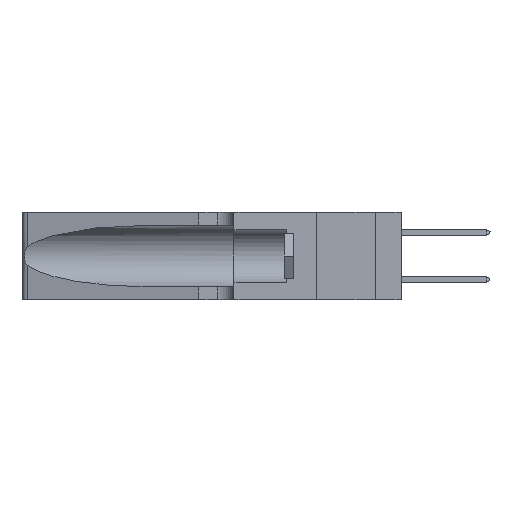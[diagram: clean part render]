
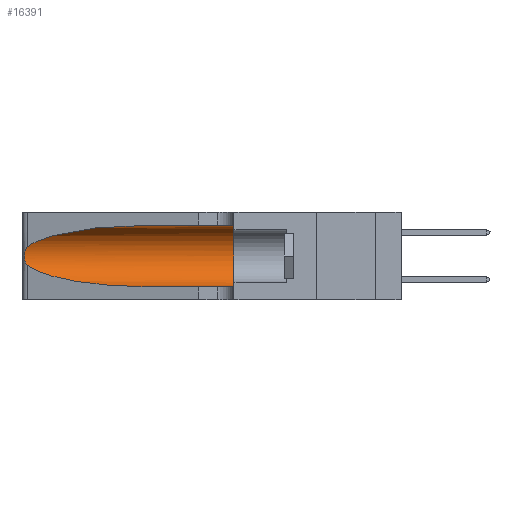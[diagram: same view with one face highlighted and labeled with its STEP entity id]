
A CAD part, left-side view. The second image highlights one B-rep face of the part: STEP entity #16391.
In plain terms, the highlighted cylindrical face has radius 3.308 mm (diameter 6.617 mm), a partial arc.
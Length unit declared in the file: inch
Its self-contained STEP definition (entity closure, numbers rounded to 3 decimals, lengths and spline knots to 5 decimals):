
#79 = DIRECTION ( 'NONE',  ( 0., 1., 0. ) ) ;
#780 = VERTEX_POINT ( 'NONE', #5503 ) ;
#1505 =( BOUNDED_CURVE ( )  B_SPLINE_CURVE ( 3, ( #8014, #35577, #5180, #27400 ),
 .UNSPECIFIED., .F., .F. ) 
 B_SPLINE_CURVE_WITH_KNOTS ( ( 4, 4 ),
 ( 1.5708, 2.84003 ),
 .UNSPECIFIED. ) 
 CURVE ( )  GEOMETRIC_REPRESENTATION_ITEM ( )  RATIONAL_B_SPLINE_CURVE ( ( 1., 0.87, 0.87, 1. ) ) 
 REPRESENTATION_ITEM ( '' )  );
#2190 = EDGE_CURVE ( 'NONE', #30342, #19642, #1505, .T. ) ;
#2523 = VERTEX_POINT ( 'NONE', #34253 ) ;
#2608 = AXIS2_PLACEMENT_3D ( 'NONE', #16649, #2687, #22255 ) ;
#2687 = DIRECTION ( 'NONE',  ( 0., -1., 0. ) ) ;
#2795 = CARTESIAN_POINT ( 'NONE',  ( 0.26075, 1.23896, 0.19203 ) ) ;
#2857 = CARTESIAN_POINT ( 'NONE',  ( 0.18966, 0.96281, 0.05475 ) ) ;
#3295 = CARTESIAN_POINT ( 'NONE',  ( 0.1305, 1.61858, 0.31525 ) ) ;
#3345 = CYLINDRICAL_SURFACE ( 'NONE', #2608, 0.13025 ) ;
#3600 = EDGE_CURVE ( 'NONE', #25010, #780, #31167, .T. ) ;
#4229 = VECTOR ( 'NONE', #25570, 39.37008 ) ;
#4769 = CARTESIAN_POINT ( 'NONE',  ( 0.1305, 0.35, 0.31525 ) ) ;
#4921 = CARTESIAN_POINT ( 'NONE',  ( 0.25854, 1.2359, 0.20912 ) ) ;
#5127 = LINE ( 'NONE', #3295, #4229 ) ;
#5180 = CARTESIAN_POINT ( 'NONE',  ( 0.2373, 1.15595, 0.28018 ) ) ;
#5503 = CARTESIAN_POINT ( 'NONE',  ( 0.1305, 0.72297, 0.05475 ) ) ;
#5655 = CARTESIAN_POINT ( 'NONE',  ( 0.26017, 1.23833, 0.17102 ) ) ;
#6719 = CARTESIAN_POINT ( 'NONE',  ( 0.1305, 1.61858, 0.05475 ) ) ;
#7642 = EDGE_CURVE ( 'NONE', #19642, #25010, #24781, .T. ) ;
#8014 = CARTESIAN_POINT ( 'NONE',  ( 0.1305, 0.72297, 0.31525 ) ) ;
#8484 = CARTESIAN_POINT ( 'NONE',  ( 0.25789, 1.23486, 0.15765 ) ) ;
#11166 = EDGE_CURVE ( 'NONE', #30342, #30793, #5127, .T. ) ;
#11323 = CARTESIAN_POINT ( 'NONE',  ( 0.25555, 1.22993, 0.14849 ) ) ;
#14020 = CARTESIAN_POINT ( 'NONE',  ( 0.25487, 1.22718, 0.14631 ) ) ;
#14827 = EDGE_LOOP ( 'NONE', ( #20320, #20358, #21930, #22823, #23377, #23722 ) ) ;
#15326 = EDGE_CURVE ( 'NONE', #780, #2523, #17873, .T. ) ;
#16123 = VECTOR ( 'NONE', #23384, 39.37008 ) ;
#16391 = ADVANCED_FACE ( 'NONE', ( #18219 ), #3345, .F. ) ;
#16649 = CARTESIAN_POINT ( 'NONE',  ( 0.1305, 1.61858, 0.185 ) ) ;
#16758 = CARTESIAN_POINT ( 'NONE',  ( 0.25787, 1.23484, 0.2124 ) ) ;
#16860 = CARTESIAN_POINT ( 'NONE',  ( 0.1305, 0.35, 0.185 ) ) ;
#17873 = LINE ( 'NONE', #6719, #16123 ) ;
#18219 = FACE_OUTER_BOUND ( 'NONE', #14827, .T. ) ;
#18977 = CARTESIAN_POINT ( 'NONE',  ( 0.25487, 1.22718, 0.14631 ) ) ;
#19562 = CARTESIAN_POINT ( 'NONE',  ( 0.26018, 1.23835, 0.19895 ) ) ;
#19642 = VERTEX_POINT ( 'NONE', #27674 ) ;
#19662 = DIRECTION ( 'NONE',  ( 0., 0., 1. ) ) ;
#19808 = CARTESIAN_POINT ( 'NONE',  ( 0.1305, 0.72297, 0.31525 ) ) ;
#20320 = ORIENTED_EDGE ( 'NONE', *, *, #2190, .T. ) ;
#20358 = ORIENTED_EDGE ( 'NONE', *, *, #7642, .T. ) ;
#21095 = AXIS2_PLACEMENT_3D ( 'NONE', #16860, #79, #19662 ) ;
#21930 = ORIENTED_EDGE ( 'NONE', *, *, #3600, .T. ) ;
#22242 = CARTESIAN_POINT ( 'NONE',  ( 0.25555, 1.22994, 0.2215 ) ) ;
#22255 = DIRECTION ( 'NONE',  ( 0., 0., -1. ) ) ;
#22353 = CARTESIAN_POINT ( 'NONE',  ( 0.26075, 1.23896, 0.178 ) ) ;
#22413 = CARTESIAN_POINT ( 'NONE',  ( 0.1305, 0.72297, 0.05475 ) ) ;
#22823 = ORIENTED_EDGE ( 'NONE', *, *, #15326, .T. ) ;
#23377 = ORIENTED_EDGE ( 'NONE', *, *, #35467, .F. ) ;
#23384 = DIRECTION ( 'NONE',  ( 0., -1., 0. ) ) ;
#23722 = ORIENTED_EDGE ( 'NONE', *, *, #11166, .F. ) ;
#24781 = B_SPLINE_CURVE_WITH_KNOTS ( 'NONE', 3,
 ( #30515, #22242, #33291, #16758, #4921, #19562, #2795, #22353, #5655, #25102, #8484, #27862, #11323, #30633 ),
 .UNSPECIFIED., .F., .F.,
 ( 4, 2, 2, 2, 2, 2, 4 ),
 ( 0., 0.00027, 0.00053, 0.00107, 0.0016, 0.00187, 0.00214 ),
 .UNSPECIFIED. ) ;
#25010 = VERTEX_POINT ( 'NONE', #18977 ) ;
#25018 = CIRCLE ( 'NONE', #21095, 0.13025 ) ;
#25102 = CARTESIAN_POINT ( 'NONE',  ( 0.25856, 1.23593, 0.16098 ) ) ;
#25570 = DIRECTION ( 'NONE',  ( 0., -1., 0. ) ) ;
#27400 = CARTESIAN_POINT ( 'NONE',  ( 0.25487, 1.22718, 0.22369 ) ) ;
#27674 = CARTESIAN_POINT ( 'NONE',  ( 0.25487, 1.22718, 0.22369 ) ) ;
#27862 = CARTESIAN_POINT ( 'NONE',  ( 0.25639, 1.23186, 0.15144 ) ) ;
#30342 = VERTEX_POINT ( 'NONE', #19808 ) ;
#30515 = CARTESIAN_POINT ( 'NONE',  ( 0.25487, 1.22718, 0.22369 ) ) ;
#30571 = CARTESIAN_POINT ( 'NONE',  ( 0.2373, 1.15595, 0.08982 ) ) ;
#30633 = CARTESIAN_POINT ( 'NONE',  ( 0.25487, 1.22718, 0.14631 ) ) ;
#30793 = VERTEX_POINT ( 'NONE', #4769 ) ;
#31167 =( BOUNDED_CURVE ( )  B_SPLINE_CURVE ( 3, ( #14020, #30571, #2857, #22413 ),
 .UNSPECIFIED., .F., .F. ) 
 B_SPLINE_CURVE_WITH_KNOTS ( ( 4, 4 ),
 ( 3.44316, 4.71239 ),
 .UNSPECIFIED. ) 
 CURVE ( )  GEOMETRIC_REPRESENTATION_ITEM ( )  RATIONAL_B_SPLINE_CURVE ( ( 1., 0.87, 0.87, 1. ) ) 
 REPRESENTATION_ITEM ( '' )  );
#33291 = CARTESIAN_POINT ( 'NONE',  ( 0.25639, 1.23184, 0.21858 ) ) ;
#34253 = CARTESIAN_POINT ( 'NONE',  ( 0.1305, 0.35, 0.05475 ) ) ;
#35467 = EDGE_CURVE ( 'NONE', #30793, #2523, #25018, .T. ) ;
#35577 = CARTESIAN_POINT ( 'NONE',  ( 0.18966, 0.96281, 0.31525 ) ) ;
